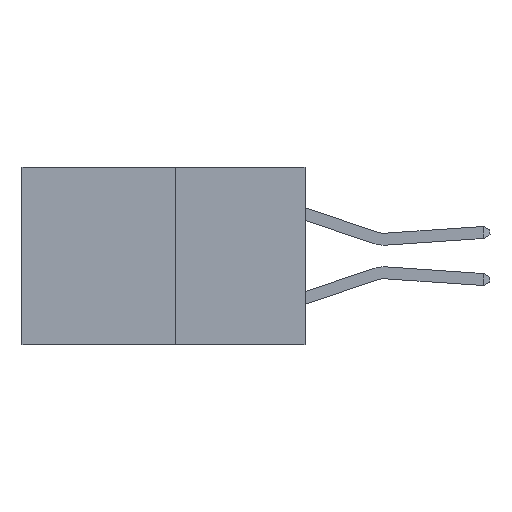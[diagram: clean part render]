
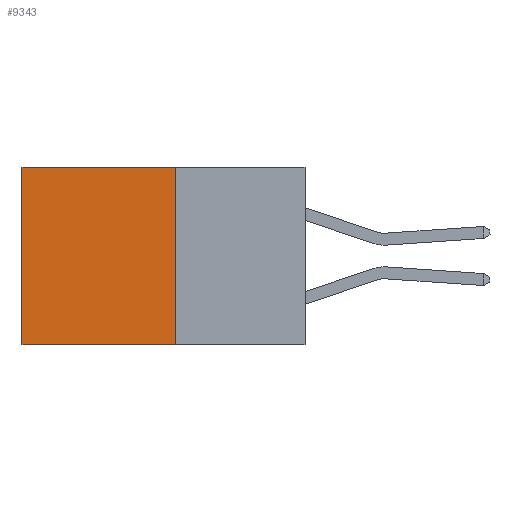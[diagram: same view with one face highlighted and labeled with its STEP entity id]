
A CAD part, left-side view. The second image highlights one B-rep face of the part: STEP entity #9343.
In plain terms, the highlighted planar face has unit normal (-1, 0, 0).
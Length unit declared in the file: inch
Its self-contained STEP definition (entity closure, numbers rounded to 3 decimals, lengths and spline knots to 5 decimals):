
#331 = CARTESIAN_POINT ( 'NONE',  ( 0.277, 0.27, -0.37 ) ) ;
#492 = CARTESIAN_POINT ( 'NONE',  ( 0.277, 0.27, -0.37 ) ) ;
#602 = CARTESIAN_POINT ( 'NONE',  ( 0.277, 0.27, 0. ) ) ;
#1305 = VERTEX_POINT ( 'NONE', #331 ) ;
#1502 = FACE_OUTER_BOUND ( 'NONE', #10350, .T. ) ;
#3262 = LINE ( 'NONE', #10610, #9935 ) ;
#4024 = CARTESIAN_POINT ( 'NONE',  ( 0.277, 0.59, 0. ) ) ;
#4575 = DIRECTION ( 'NONE',  ( 0., 1., 0. ) ) ;
#4589 = CARTESIAN_POINT ( 'NONE',  ( 0.277, 0.59, -0.37 ) ) ;
#4669 = EDGE_CURVE ( 'NONE', #9790, #5129, #4946, .T. ) ;
#4822 = EDGE_CURVE ( 'NONE', #5129, #6209, #6185, .T. ) ;
#4847 = CARTESIAN_POINT ( 'NONE',  ( 0.277, 0.27, -0.37 ) ) ;
#4946 = LINE ( 'NONE', #6217, #9312 ) ;
#5129 = VERTEX_POINT ( 'NONE', #4024 ) ;
#5156 = ORIENTED_EDGE ( 'NONE', *, *, #6176, .F. ) ;
#5774 = CARTESIAN_POINT ( 'NONE',  ( 0.277, 0.59, -0.37 ) ) ;
#5821 = EDGE_CURVE ( 'NONE', #1305, #6209, #3262, .T. ) ;
#6176 = EDGE_CURVE ( 'NONE', #9790, #1305, #10326, .T. ) ;
#6185 = LINE ( 'NONE', #4589, #10461 ) ;
#6209 = VERTEX_POINT ( 'NONE', #5774 ) ;
#6217 = CARTESIAN_POINT ( 'NONE',  ( 0.277, 0.27, 0. ) ) ;
#6358 = DIRECTION ( 'NONE',  ( 0., 0., -1. ) ) ;
#6420 = ORIENTED_EDGE ( 'NONE', *, *, #4822, .T. ) ;
#7742 = ORIENTED_EDGE ( 'NONE', *, *, #5821, .F. ) ;
#7882 = DIRECTION ( 'NONE',  ( 0., 0., -1. ) ) ;
#8098 = VECTOR ( 'NONE', #8404, 39.37008 ) ;
#8404 = DIRECTION ( 'NONE',  ( 0., 0., -1. ) ) ;
#8913 = ORIENTED_EDGE ( 'NONE', *, *, #4669, .T. ) ;
#9235 = AXIS2_PLACEMENT_3D ( 'NONE', #492, #10368, #7882 ) ;
#9312 = VECTOR ( 'NONE', #11293, 39.37008 ) ;
#9343 = ADVANCED_FACE ( 'NONE', ( #1502 ), #11201, .F. ) ;
#9790 = VERTEX_POINT ( 'NONE', #602 ) ;
#9935 = VECTOR ( 'NONE', #4575, 39.37008 ) ;
#10326 = LINE ( 'NONE', #4847, #8098 ) ;
#10350 = EDGE_LOOP ( 'NONE', ( #6420, #7742, #5156, #8913 ) ) ;
#10368 = DIRECTION ( 'NONE',  ( 1., 0., 0. ) ) ;
#10461 = VECTOR ( 'NONE', #6358, 39.37008 ) ;
#10610 = CARTESIAN_POINT ( 'NONE',  ( 0.277, 0.27, -0.37 ) ) ;
#11201 = PLANE ( 'NONE',  #9235 ) ;
#11293 = DIRECTION ( 'NONE',  ( 0., 1., 0. ) ) ;
